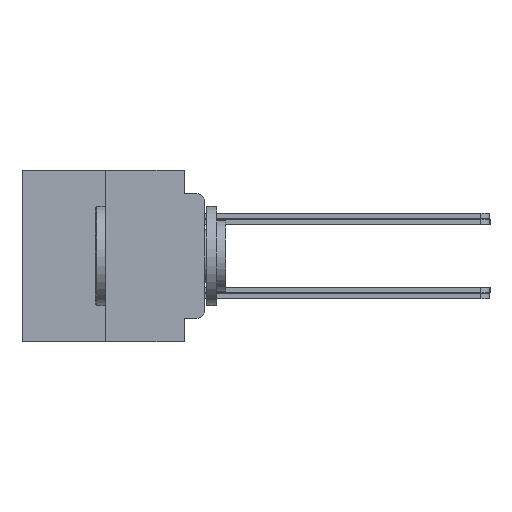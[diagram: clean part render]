
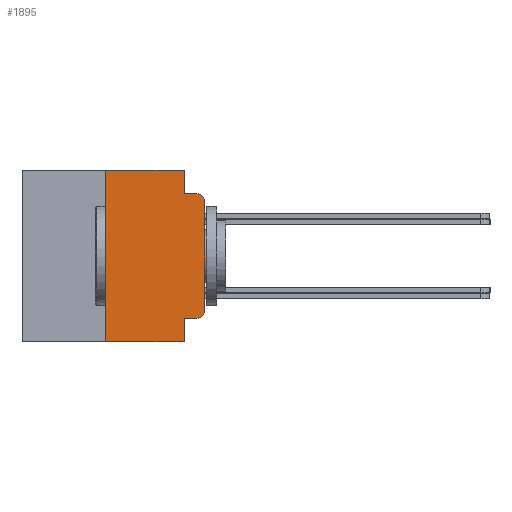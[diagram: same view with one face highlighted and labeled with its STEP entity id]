
A CAD part, left-side view. The second image highlights one B-rep face of the part: STEP entity #1895.
In plain terms, the highlighted planar face has unit normal (-1, 0, 0).
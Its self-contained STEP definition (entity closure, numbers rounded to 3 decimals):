
#60 = EDGE_CURVE ( 'NONE', #21072, #23321, #18227, .T. ) ;
#430 = ORIENTED_EDGE ( 'NONE', *, *, #60, .T. ) ;
#626 = DIRECTION ( 'NONE',  ( 0., -1., 0. ) ) ;
#706 = VERTEX_POINT ( 'NONE', #888 ) ;
#709 = VECTOR ( 'NONE', #28654, 1000. ) ;
#888 = CARTESIAN_POINT ( 'NONE',  ( -75.603, 1.295, 3.975 ) ) ;
#916 = DIRECTION ( 'NONE',  ( 0., 0., 1. ) ) ;
#1126 = ORIENTED_EDGE ( 'NONE', *, *, #1551, .T. ) ;
#1266 = CARTESIAN_POINT ( 'NONE',  ( -75.603, 11.684, -5.486 ) ) ;
#1326 = EDGE_CURVE ( 'NONE', #20144, #13892, #4570, .T. ) ;
#1551 = EDGE_CURVE ( 'NONE', #23321, #2838, #24579, .T. ) ;
#1895 = ADVANCED_FACE ( 'NONE', ( #10966 ), #3262, .F. ) ;
#2838 = VERTEX_POINT ( 'NONE', #12744 ) ;
#2840 = VECTOR ( 'NONE', #5210, 1000. ) ;
#3195 = LINE ( 'NONE', #1266, #709 ) ;
#3260 = AXIS2_PLACEMENT_3D ( 'NONE', #12546, #12448, #10536 ) ;
#3262 = PLANE ( 'NONE',  #23791 ) ;
#3408 = VERTEX_POINT ( 'NONE', #15714 ) ;
#3680 = CARTESIAN_POINT ( 'NONE',  ( -75.603, 1.295, -3.975 ) ) ;
#4570 = LINE ( 'NONE', #9684, #8474 ) ;
#4818 = EDGE_CURVE ( 'NONE', #16394, #20144, #8284, .T. ) ;
#5210 = DIRECTION ( 'NONE',  ( 0., -1., 0. ) ) ;
#5638 = CIRCLE ( 'NONE', #3260, 0.508 ) ;
#6950 = CARTESIAN_POINT ( 'NONE',  ( -75.603, 6.35, -5.486 ) ) ;
#7584 = ORIENTED_EDGE ( 'NONE', *, *, #12660, .T. ) ;
#7664 = VERTEX_POINT ( 'NONE', #25804 ) ;
#7877 = CARTESIAN_POINT ( 'NONE',  ( -75.603, 0., 3.467 ) ) ;
#8083 = VECTOR ( 'NONE', #22589, 1000. ) ;
#8164 = ORIENTED_EDGE ( 'NONE', *, *, #17667, .T. ) ;
#8284 = LINE ( 'NONE', #16809, #15473 ) ;
#8474 = VECTOR ( 'NONE', #626, 1000. ) ;
#8477 = EDGE_LOOP ( 'NONE', ( #430, #1126, #8164, #7584, #11978, #26969, #18964, #23166, #13321, #9000 ) ) ;
#9000 = ORIENTED_EDGE ( 'NONE', *, *, #28031, .F. ) ;
#9132 = LINE ( 'NONE', #15603, #8083 ) ;
#9530 = DIRECTION ( 'NONE',  ( 0., -1., 0. ) ) ;
#9683 = CARTESIAN_POINT ( 'NONE',  ( -75.603, 1.295, -3.975 ) ) ;
#9684 = CARTESIAN_POINT ( 'NONE',  ( -75.603, 11.684, 5.486 ) ) ;
#9953 = DIRECTION ( 'NONE',  ( 0., 0., -1. ) ) ;
#10425 = LINE ( 'NONE', #25637, #15821 ) ;
#10536 = DIRECTION ( 'NONE',  ( 0., 0., -1. ) ) ;
#10593 = EDGE_CURVE ( 'NONE', #706, #3408, #10425, .T. ) ;
#10692 = VECTOR ( 'NONE', #10896, 1000. ) ;
#10896 = DIRECTION ( 'NONE',  ( 0., 0., -1. ) ) ;
#10966 = FACE_OUTER_BOUND ( 'NONE', #8477, .T. ) ;
#11179 = CARTESIAN_POINT ( 'NONE',  ( -75.603, 1.295, 5.486 ) ) ;
#11666 = EDGE_CURVE ( 'NONE', #13892, #706, #25356, .T. ) ;
#11978 = ORIENTED_EDGE ( 'NONE', *, *, #10593, .F. ) ;
#12448 = DIRECTION ( 'NONE',  ( -1., 0., 0. ) ) ;
#12546 = CARTESIAN_POINT ( 'NONE',  ( -75.603, 0.508, 3.467 ) ) ;
#12660 = EDGE_CURVE ( 'NONE', #13634, #3408, #5638, .T. ) ;
#12744 = CARTESIAN_POINT ( 'NONE',  ( -75.603, 0., -3.467 ) ) ;
#13321 = ORIENTED_EDGE ( 'NONE', *, *, #21580, .T. ) ;
#13634 = VERTEX_POINT ( 'NONE', #7877 ) ;
#13892 = VERTEX_POINT ( 'NONE', #11179 ) ;
#15473 = VECTOR ( 'NONE', #916, 1000. ) ;
#15603 = CARTESIAN_POINT ( 'NONE',  ( -75.603, 1.295, 0. ) ) ;
#15714 = CARTESIAN_POINT ( 'NONE',  ( -75.603, 0.508, 3.975 ) ) ;
#15739 = LINE ( 'NONE', #24133, #24344 ) ;
#15821 = VECTOR ( 'NONE', #9530, 1000. ) ;
#16394 = VERTEX_POINT ( 'NONE', #6950 ) ;
#16809 = CARTESIAN_POINT ( 'NONE',  ( -75.603, 6.35, -5.486 ) ) ;
#16842 = AXIS2_PLACEMENT_3D ( 'NONE', #29010, #17506, #22214 ) ;
#17506 = DIRECTION ( 'NONE',  ( -1., 0., 0. ) ) ;
#17512 = DIRECTION ( 'NONE',  ( 0., 0., 1. ) ) ;
#17667 = EDGE_CURVE ( 'NONE', #2838, #13634, #15739, .T. ) ;
#18227 = LINE ( 'NONE', #9683, #2840 ) ;
#18964 = ORIENTED_EDGE ( 'NONE', *, *, #1326, .F. ) ;
#19923 = CARTESIAN_POINT ( 'NONE',  ( -75.603, 1.295, 0. ) ) ;
#20144 = VERTEX_POINT ( 'NONE', #25932 ) ;
#21072 = VERTEX_POINT ( 'NONE', #3680 ) ;
#21501 = CARTESIAN_POINT ( 'NONE',  ( -75.603, 0.508, -3.975 ) ) ;
#21580 = EDGE_CURVE ( 'NONE', #16394, #7664, #3195, .T. ) ;
#22214 = DIRECTION ( 'NONE',  ( 0., 0., -1. ) ) ;
#22589 = DIRECTION ( 'NONE',  ( 0., 0., -1. ) ) ;
#23166 = ORIENTED_EDGE ( 'NONE', *, *, #4818, .F. ) ;
#23321 = VERTEX_POINT ( 'NONE', #21501 ) ;
#23791 = AXIS2_PLACEMENT_3D ( 'NONE', #27964, #28272, #9953 ) ;
#24133 = CARTESIAN_POINT ( 'NONE',  ( -75.603, 0., 5.486 ) ) ;
#24344 = VECTOR ( 'NONE', #17512, 1000. ) ;
#24579 = CIRCLE ( 'NONE', #16842, 0.508 ) ;
#25356 = LINE ( 'NONE', #19923, #10692 ) ;
#25637 = CARTESIAN_POINT ( 'NONE',  ( -75.603, 1.295, 3.975 ) ) ;
#25804 = CARTESIAN_POINT ( 'NONE',  ( -75.603, 1.295, -5.486 ) ) ;
#25932 = CARTESIAN_POINT ( 'NONE',  ( -75.603, 6.35, 5.486 ) ) ;
#26969 = ORIENTED_EDGE ( 'NONE', *, *, #11666, .F. ) ;
#27964 = CARTESIAN_POINT ( 'NONE',  ( -75.603, 11.684, 5.486 ) ) ;
#28031 = EDGE_CURVE ( 'NONE', #21072, #7664, #9132, .T. ) ;
#28272 = DIRECTION ( 'NONE',  ( 1., 0., 0. ) ) ;
#28654 = DIRECTION ( 'NONE',  ( 0., -1., 0. ) ) ;
#29010 = CARTESIAN_POINT ( 'NONE',  ( -75.603, 0.508, -3.467 ) ) ;
